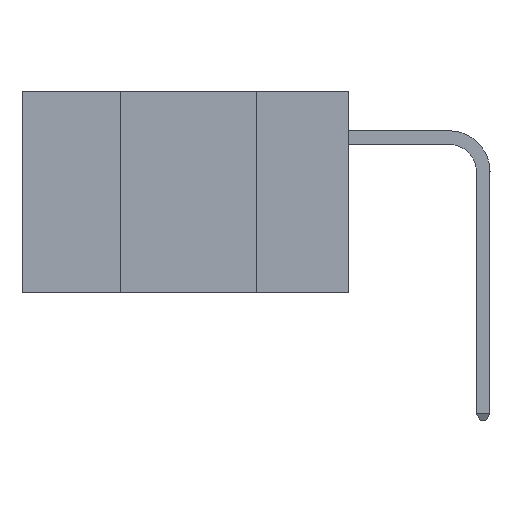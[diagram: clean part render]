
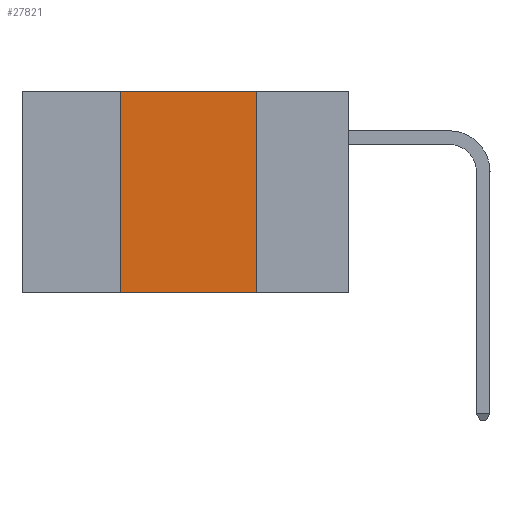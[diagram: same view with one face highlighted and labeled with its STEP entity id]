
A CAD part, left-side view. The second image highlights one B-rep face of the part: STEP entity #27821.
In plain terms, the highlighted planar face has unit normal (-1, 0, 0).
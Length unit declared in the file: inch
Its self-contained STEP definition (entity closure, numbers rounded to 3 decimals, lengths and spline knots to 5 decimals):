
#823 = DIRECTION ( 'NONE',  ( 0., 0., -1. ) ) ;
#1965 = LINE ( 'NONE', #23757, #14376 ) ;
#3122 = DIRECTION ( 'NONE',  ( 0., -1., 0. ) ) ;
#3435 = ORIENTED_EDGE ( 'NONE', *, *, #30671, .F. ) ;
#3512 = DIRECTION ( 'NONE',  ( 0., 0., 1. ) ) ;
#5709 = CARTESIAN_POINT ( 'NONE',  ( 0., 0.42, 0. ) ) ;
#7375 = VERTEX_POINT ( 'NONE', #26597 ) ;
#8546 = FACE_OUTER_BOUND ( 'NONE', #15773, .T. ) ;
#9415 = LINE ( 'NONE', #11913, #32133 ) ;
#11047 = LINE ( 'NONE', #26752, #18960 ) ;
#11257 = EDGE_CURVE ( 'NONE', #30745, #7375, #30820, .T. ) ;
#11913 = CARTESIAN_POINT ( 'NONE',  ( 0., 0.42, 0. ) ) ;
#12282 = ORIENTED_EDGE ( 'NONE', *, *, #28390, .F. ) ;
#14376 = VECTOR ( 'NONE', #34674, 39.37008 ) ;
#15355 = ORIENTED_EDGE ( 'NONE', *, *, #28946, .F. ) ;
#15773 = EDGE_LOOP ( 'NONE', ( #12282, #15355, #3435, #16170 ) ) ;
#16170 = ORIENTED_EDGE ( 'NONE', *, *, #11257, .T. ) ;
#16617 = VECTOR ( 'NONE', #3122, 39.37008 ) ;
#17656 = VERTEX_POINT ( 'NONE', #5709 ) ;
#18960 = VECTOR ( 'NONE', #34994, 39.37008 ) ;
#22231 = CARTESIAN_POINT ( 'NONE',  ( 0., 0.6, -0.37 ) ) ;
#23175 = CARTESIAN_POINT ( 'NONE',  ( 0., 0.17, 0. ) ) ;
#23757 = CARTESIAN_POINT ( 'NONE',  ( 0., 0.17, 0. ) ) ;
#24772 = CARTESIAN_POINT ( 'NONE',  ( 0., 0.6, 0. ) ) ;
#25299 = PLANE ( 'NONE',  #30913 ) ;
#26597 = CARTESIAN_POINT ( 'NONE',  ( 0., 0.17, -0.37 ) ) ;
#26752 = CARTESIAN_POINT ( 'NONE',  ( 0., 0.6, 0. ) ) ;
#27507 = VERTEX_POINT ( 'NONE', #23175 ) ;
#27821 = ADVANCED_FACE ( 'NONE', ( #8546 ), #25299, .F. ) ;
#28390 = EDGE_CURVE ( 'NONE', #27507, #7375, #1965, .T. ) ;
#28946 = EDGE_CURVE ( 'NONE', #17656, #27507, #11047, .T. ) ;
#30671 = EDGE_CURVE ( 'NONE', #30745, #17656, #9415, .T. ) ;
#30745 = VERTEX_POINT ( 'NONE', #34410 ) ;
#30820 = LINE ( 'NONE', #22231, #16617 ) ;
#30913 = AXIS2_PLACEMENT_3D ( 'NONE', #24772, #33014, #823 ) ;
#32133 = VECTOR ( 'NONE', #3512, 39.37008 ) ;
#33014 = DIRECTION ( 'NONE',  ( 1., 0., 0. ) ) ;
#34410 = CARTESIAN_POINT ( 'NONE',  ( 0., 0.42, -0.37 ) ) ;
#34674 = DIRECTION ( 'NONE',  ( 0., 0., -1. ) ) ;
#34994 = DIRECTION ( 'NONE',  ( 0., -1., 0. ) ) ;
